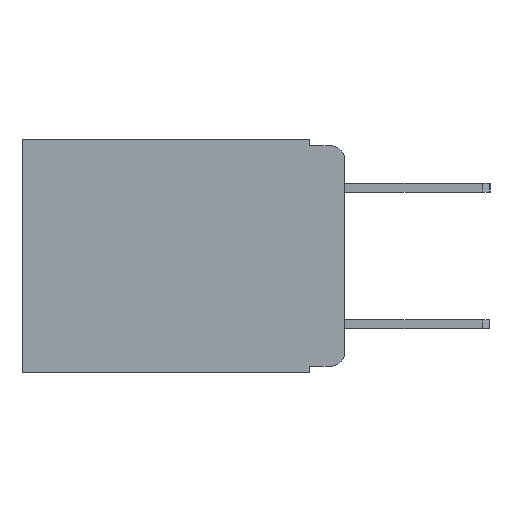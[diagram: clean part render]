
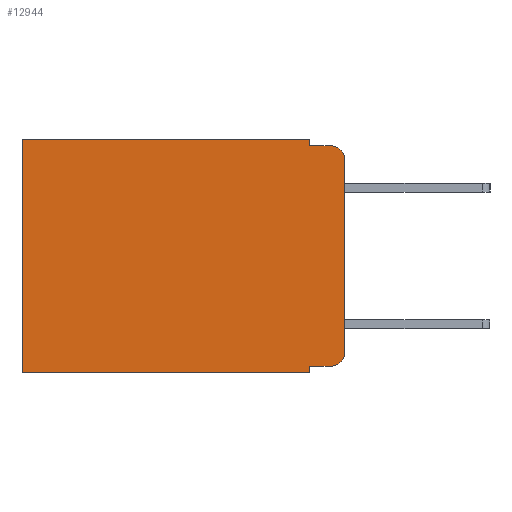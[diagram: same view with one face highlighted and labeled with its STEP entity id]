
A CAD part, left-side view. The second image highlights one B-rep face of the part: STEP entity #12944.
In plain terms, the highlighted planar face has unit normal (-1, 0, 0).
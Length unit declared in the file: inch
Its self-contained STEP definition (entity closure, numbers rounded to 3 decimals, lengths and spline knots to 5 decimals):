
#60 = DIRECTION ( 'NONE',  ( 0., 0., -1. ) ) ;
#171 = CARTESIAN_POINT ( 'NONE',  ( 0.298, 0.051, -0.01 ) ) ;
#202 = DIRECTION ( 'NONE',  ( 0., -1., 0. ) ) ;
#312 = LINE ( 'NONE', #565, #16623 ) ;
#441 = DIRECTION ( 'NONE',  ( 0., 0., -1. ) ) ;
#565 = CARTESIAN_POINT ( 'NONE',  ( 0.298, 0., 0. ) ) ;
#611 = VECTOR ( 'NONE', #11658, 39.37008 ) ;
#653 = VERTEX_POINT ( 'NONE', #10953 ) ;
#765 = CARTESIAN_POINT ( 'NONE',  ( 0.298, 0.02, -0.01 ) ) ;
#923 = VECTOR ( 'NONE', #5201, 39.37008 ) ;
#2034 = VERTEX_POINT ( 'NONE', #18601 ) ;
#2129 = AXIS2_PLACEMENT_3D ( 'NONE', #12260, #9430, #9104 ) ;
#2267 = DIRECTION ( 'NONE',  ( 0., 0., -1. ) ) ;
#2535 = ORIENTED_EDGE ( 'NONE', *, *, #9246, .T. ) ;
#2885 = LINE ( 'NONE', #9754, #18909 ) ;
#2896 = EDGE_CURVE ( 'NONE', #3114, #17064, #14485, .T. ) ;
#2925 = EDGE_CURVE ( 'NONE', #13402, #9478, #6198, .T. ) ;
#3114 = VERTEX_POINT ( 'NONE', #9030 ) ;
#3533 = CIRCLE ( 'NONE', #8509, 0.02 ) ;
#4059 = EDGE_CURVE ( 'NONE', #5279, #10616, #10401, .T. ) ;
#4743 = LINE ( 'NONE', #8346, #923 ) ;
#4903 = CARTESIAN_POINT ( 'NONE',  ( 0.298, 0.051, 0. ) ) ;
#5201 = DIRECTION ( 'NONE',  ( 0., 1., 0. ) ) ;
#5279 = VERTEX_POINT ( 'NONE', #9252 ) ;
#5300 = ORIENTED_EDGE ( 'NONE', *, *, #9988, .F. ) ;
#6198 = CIRCLE ( 'NONE', #2129, 0.02 ) ;
#6272 = ORIENTED_EDGE ( 'NONE', *, *, #17524, .T. ) ;
#6533 = LINE ( 'NONE', #4903, #18330 ) ;
#7062 = ORIENTED_EDGE ( 'NONE', *, *, #17381, .F. ) ;
#8186 = CARTESIAN_POINT ( 'NONE',  ( 0.298, 0.02, -0.333 ) ) ;
#8346 = CARTESIAN_POINT ( 'NONE',  ( 0.298, 0., 0. ) ) ;
#8509 = AXIS2_PLACEMENT_3D ( 'NONE', #19189, #10121, #441 ) ;
#8540 = DIRECTION ( 'NONE',  ( 0., 0., -1. ) ) ;
#9030 = CARTESIAN_POINT ( 'NONE',  ( 0.298, 0.051, -0.01 ) ) ;
#9037 = ORIENTED_EDGE ( 'NONE', *, *, #2896, .F. ) ;
#9104 = DIRECTION ( 'NONE',  ( 0., 0., -1. ) ) ;
#9246 = EDGE_CURVE ( 'NONE', #2034, #12274, #4743, .T. ) ;
#9252 = CARTESIAN_POINT ( 'NONE',  ( 0.298, 0.051, -0.343 ) ) ;
#9430 = DIRECTION ( 'NONE',  ( -1., 0., 0. ) ) ;
#9478 = VERTEX_POINT ( 'NONE', #19569 ) ;
#9547 = ORIENTED_EDGE ( 'NONE', *, *, #2925, .T. ) ;
#9697 = DIRECTION ( 'NONE',  ( 0., 0., -1. ) ) ;
#9754 = CARTESIAN_POINT ( 'NONE',  ( 0.298, 0.473, 0. ) ) ;
#9988 = EDGE_CURVE ( 'NONE', #2034, #3114, #16872, .T. ) ;
#10121 = DIRECTION ( 'NONE',  ( -1., 0., 0. ) ) ;
#10171 = CARTESIAN_POINT ( 'NONE',  ( 0.298, 0., -0.343 ) ) ;
#10401 = LINE ( 'NONE', #10171, #13964 ) ;
#10465 = CARTESIAN_POINT ( 'NONE',  ( 0.298, 0.051, -0.333 ) ) ;
#10616 = VERTEX_POINT ( 'NONE', #11571 ) ;
#10759 = DIRECTION ( 'NONE',  ( 0., -1., 0. ) ) ;
#10953 = CARTESIAN_POINT ( 'NONE',  ( 0.298, 0., -0.03 ) ) ;
#11389 = VECTOR ( 'NONE', #202, 39.37008 ) ;
#11571 = CARTESIAN_POINT ( 'NONE',  ( 0.298, 0.473, -0.343 ) ) ;
#11658 = DIRECTION ( 'NONE',  ( 0., 0., -1. ) ) ;
#11798 = EDGE_CURVE ( 'NONE', #12274, #10616, #2885, .T. ) ;
#12163 = ORIENTED_EDGE ( 'NONE', *, *, #20103, .F. ) ;
#12260 = CARTESIAN_POINT ( 'NONE',  ( 0.298, 0.02, -0.313 ) ) ;
#12274 = VERTEX_POINT ( 'NONE', #19098 ) ;
#12682 = LINE ( 'NONE', #18335, #20182 ) ;
#12850 = EDGE_LOOP ( 'NONE', ( #12163, #6272, #9037, #5300, #2535, #12900, #17420, #7062, #19733, #9547 ) ) ;
#12900 = ORIENTED_EDGE ( 'NONE', *, *, #11798, .T. ) ;
#12944 = ADVANCED_FACE ( 'NONE', ( #15359 ), #13126, .F. ) ;
#13126 = PLANE ( 'NONE',  #14648 ) ;
#13402 = VERTEX_POINT ( 'NONE', #8186 ) ;
#13714 = EDGE_CURVE ( 'NONE', #19089, #13402, #12682, .T. ) ;
#13964 = VECTOR ( 'NONE', #18663, 39.37008 ) ;
#14485 = LINE ( 'NONE', #171, #11389 ) ;
#14648 = AXIS2_PLACEMENT_3D ( 'NONE', #16199, #17697, #8540 ) ;
#15359 = FACE_OUTER_BOUND ( 'NONE', #12850, .T. ) ;
#16199 = CARTESIAN_POINT ( 'NONE',  ( 0.298, 0., 0. ) ) ;
#16623 = VECTOR ( 'NONE', #2267, 39.37008 ) ;
#16872 = LINE ( 'NONE', #17743, #611 ) ;
#17064 = VERTEX_POINT ( 'NONE', #765 ) ;
#17381 = EDGE_CURVE ( 'NONE', #19089, #5279, #6533, .T. ) ;
#17420 = ORIENTED_EDGE ( 'NONE', *, *, #4059, .F. ) ;
#17524 = EDGE_CURVE ( 'NONE', #653, #17064, #3533, .T. ) ;
#17697 = DIRECTION ( 'NONE',  ( 1., 0., 0. ) ) ;
#17743 = CARTESIAN_POINT ( 'NONE',  ( 0.298, 0.051, 0. ) ) ;
#18330 = VECTOR ( 'NONE', #9697, 39.37008 ) ;
#18335 = CARTESIAN_POINT ( 'NONE',  ( 0.298, 0.051, -0.333 ) ) ;
#18601 = CARTESIAN_POINT ( 'NONE',  ( 0.298, 0.051, 0. ) ) ;
#18663 = DIRECTION ( 'NONE',  ( 0., 1., 0. ) ) ;
#18909 = VECTOR ( 'NONE', #60, 39.37008 ) ;
#19089 = VERTEX_POINT ( 'NONE', #10465 ) ;
#19098 = CARTESIAN_POINT ( 'NONE',  ( 0.298, 0.473, 0. ) ) ;
#19189 = CARTESIAN_POINT ( 'NONE',  ( 0.298, 0.02, -0.03 ) ) ;
#19569 = CARTESIAN_POINT ( 'NONE',  ( 0.298, 0., -0.313 ) ) ;
#19733 = ORIENTED_EDGE ( 'NONE', *, *, #13714, .T. ) ;
#20103 = EDGE_CURVE ( 'NONE', #653, #9478, #312, .T. ) ;
#20182 = VECTOR ( 'NONE', #10759, 39.37008 ) ;
